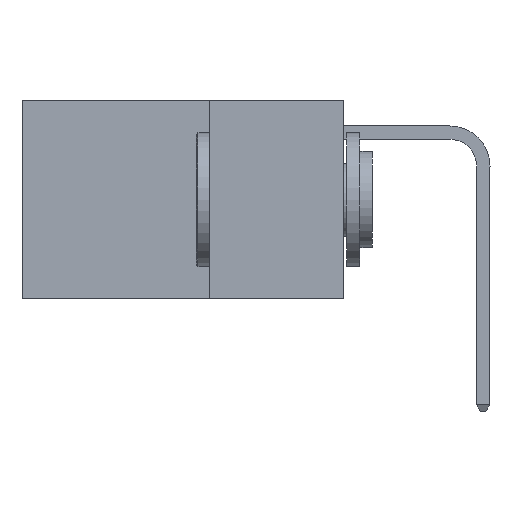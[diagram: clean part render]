
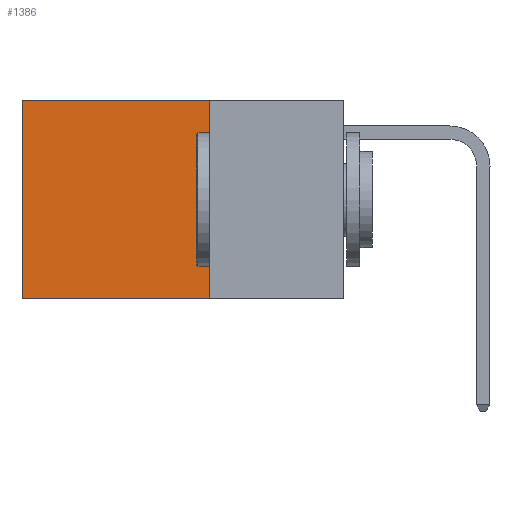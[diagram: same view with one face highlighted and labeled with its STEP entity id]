
A CAD part, left-side view. The second image highlights one B-rep face of the part: STEP entity #1386.
In plain terms, the highlighted planar face has unit normal (-1, 0, 0).
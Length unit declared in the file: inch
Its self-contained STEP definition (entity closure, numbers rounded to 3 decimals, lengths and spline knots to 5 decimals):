
#254 = ORIENTED_EDGE ( 'NONE', *, *, #21116, .F. ) ;
#1386 = ADVANCED_FACE ( 'NONE', ( #25487 ), #23301, .F. ) ;
#1885 = VECTOR ( 'NONE', #17199, 39.37008 ) ;
#2333 = VECTOR ( 'NONE', #21410, 39.37008 ) ;
#2546 = ORIENTED_EDGE ( 'NONE', *, *, #22226, .T. ) ;
#2694 = CARTESIAN_POINT ( 'NONE',  ( 0.2625, 0.25, -0.37 ) ) ;
#3012 = LINE ( 'NONE', #15256, #2333 ) ;
#3214 = LINE ( 'NONE', #15086, #1885 ) ;
#3469 = VERTEX_POINT ( 'NONE', #15554 ) ;
#5760 = LINE ( 'NONE', #15566, #22521 ) ;
#7647 = EDGE_CURVE ( 'NONE', #9571, #3469, #5760, .T. ) ;
#9146 = DIRECTION ( 'NONE',  ( 0., 0., -1. ) ) ;
#9571 = VERTEX_POINT ( 'NONE', #19841 ) ;
#10111 = ORIENTED_EDGE ( 'NONE', *, *, #7647, .T. ) ;
#15086 = CARTESIAN_POINT ( 'NONE',  ( 0.2625, 0.25, 0. ) ) ;
#15256 = CARTESIAN_POINT ( 'NONE',  ( 0.2625, 0.25, 0. ) ) ;
#15554 = CARTESIAN_POINT ( 'NONE',  ( 0.2625, 0.6, -0.37 ) ) ;
#15566 = CARTESIAN_POINT ( 'NONE',  ( 0.2625, 0.6, 0. ) ) ;
#17199 = DIRECTION ( 'NONE',  ( 0., 0., -1. ) ) ;
#17396 = EDGE_CURVE ( 'NONE', #23782, #18228, #3214, .T. ) ;
#18228 = VERTEX_POINT ( 'NONE', #24786 ) ;
#19841 = CARTESIAN_POINT ( 'NONE',  ( 0.2625, 0.6, 0. ) ) ;
#20249 = CARTESIAN_POINT ( 'NONE',  ( 0.2625, 0.25, 0. ) ) ;
#21116 = EDGE_CURVE ( 'NONE', #18228, #3469, #21592, .T. ) ;
#21177 = ORIENTED_EDGE ( 'NONE', *, *, #17396, .F. ) ;
#21410 = DIRECTION ( 'NONE',  ( 0., 1., 0. ) ) ;
#21592 = LINE ( 'NONE', #2694, #25795 ) ;
#22226 = EDGE_CURVE ( 'NONE', #23782, #9571, #3012, .T. ) ;
#22521 = VECTOR ( 'NONE', #9146, 39.37008 ) ;
#23210 = DIRECTION ( 'NONE',  ( 0., 0., -1. ) ) ;
#23243 = DIRECTION ( 'NONE',  ( 1., 0., 0. ) ) ;
#23282 = CARTESIAN_POINT ( 'NONE',  ( 0.2625, 0.25, 0. ) ) ;
#23301 = PLANE ( 'NONE',  #24862 ) ;
#23695 = DIRECTION ( 'NONE',  ( 0., 1., 0. ) ) ;
#23782 = VERTEX_POINT ( 'NONE', #20249 ) ;
#24786 = CARTESIAN_POINT ( 'NONE',  ( 0.2625, 0.25, -0.37 ) ) ;
#24862 = AXIS2_PLACEMENT_3D ( 'NONE', #23282, #23243, #23210 ) ;
#25487 = FACE_OUTER_BOUND ( 'NONE', #25972, .T. ) ;
#25795 = VECTOR ( 'NONE', #23695, 39.37008 ) ;
#25972 = EDGE_LOOP ( 'NONE', ( #10111, #254, #21177, #2546 ) ) ;
